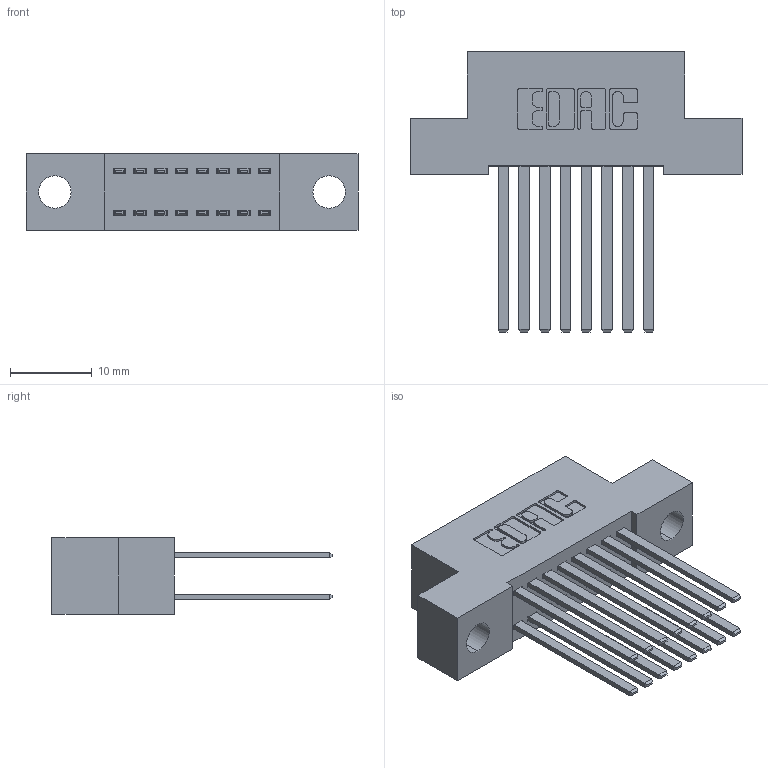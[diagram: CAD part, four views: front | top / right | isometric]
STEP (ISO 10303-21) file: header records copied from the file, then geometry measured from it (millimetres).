
FILE_DESCRIPTION (( 'STEP AP203' ), '1' );
FILE_NAME ('342-016-544-204.STEP', '2019-10-01T19:03:07', ( '' ), ( '' ), 'SwSTEP 2.0', 'SolidWorks 2016', '' );
FILE_SCHEMA (( 'CONFIG_CONTROL_DESIGN' ));
Length unit declared in the file: inch
Products named in the file (3): 342 Part_.156 TH; 345-292-001_345-293-144; 342-016-544-204
Assembly tree (17 placements, depth 2):
  342-016-544-204
    342 Part_.156 TH
    345-292-001_345-293-144  x16
Bounding box: 40.64 x 34.3 x 9.4 mm (x, y, z)
Volume: 3627.8 mm3; surface area: 5512.8 mm2
Topology: 17 solids, 17 shells, 846 faces, 2491 edges, 1638 vertices
Faces by surface type: plane 578, cylinder 268
Entity records: 9231 total; most frequent: CARTESIAN_POINT 1566, ORIENTED_EDGE 1502, DIRECTION 1395, EDGE_CURVE 751, VECTOR 627, LINE 627, VERTEX_POINT 498, AXIS2_PLACEMENT_3D 384
